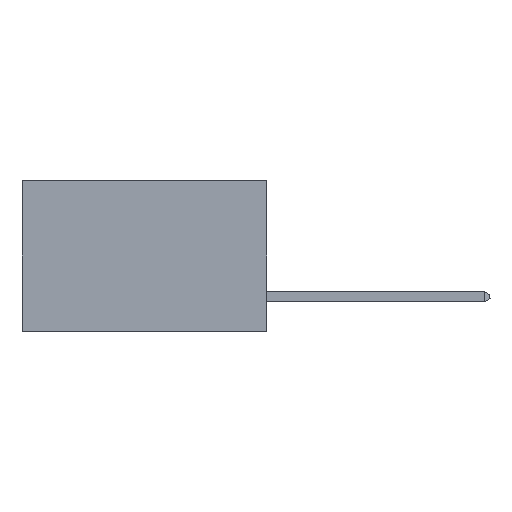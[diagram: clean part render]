
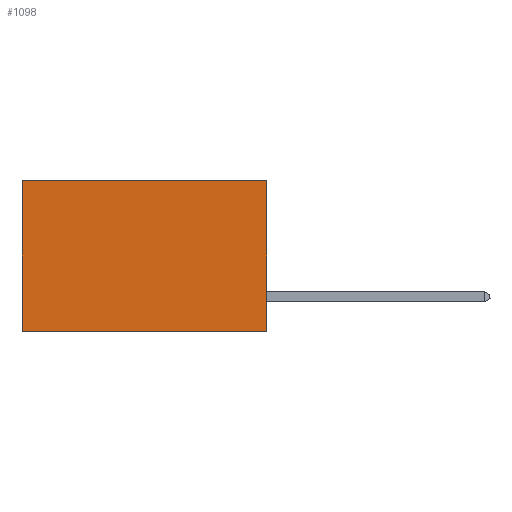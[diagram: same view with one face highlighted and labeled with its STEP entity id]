
A CAD part, left-side view. The second image highlights one B-rep face of the part: STEP entity #1098.
In plain terms, the highlighted planar face has unit normal (-1, 0, 0).
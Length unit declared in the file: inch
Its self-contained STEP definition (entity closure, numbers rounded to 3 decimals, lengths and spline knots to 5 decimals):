
#548 = LINE ( 'NONE', #18708, #14343 ) ;
#1098 = ADVANCED_FACE ( 'NONE', ( #4357 ), #11884, .F. ) ;
#1171 = VERTEX_POINT ( 'NONE', #11953 ) ;
#1679 = EDGE_CURVE ( 'NONE', #11081, #1171, #4578, .T. ) ;
#2158 = CARTESIAN_POINT ( 'NONE',  ( 0.2875, 0., -0.37 ) ) ;
#2663 = VECTOR ( 'NONE', #13475, 39.37008 ) ;
#3350 = VERTEX_POINT ( 'NONE', #3455 ) ;
#3455 = CARTESIAN_POINT ( 'NONE',  ( 0.2875, 0.6, 0. ) ) ;
#3482 = DIRECTION ( 'NONE',  ( 0., 1., 0. ) ) ;
#4357 = FACE_OUTER_BOUND ( 'NONE', #10040, .T. ) ;
#4578 = LINE ( 'NONE', #5097, #11455 ) ;
#5021 = VECTOR ( 'NONE', #8514, 39.37008 ) ;
#5097 = CARTESIAN_POINT ( 'NONE',  ( 0.2875, 0., -0.37 ) ) ;
#6683 = CARTESIAN_POINT ( 'NONE',  ( 0.2875, 0., 0. ) ) ;
#8136 = LINE ( 'NONE', #19115, #5021 ) ;
#8514 = DIRECTION ( 'NONE',  ( 0., 1., 0. ) ) ;
#10040 = EDGE_LOOP ( 'NONE', ( #17172, #18937, #10518, #14161 ) ) ;
#10326 = AXIS2_PLACEMENT_3D ( 'NONE', #10358, #12017, #13566 ) ;
#10358 = CARTESIAN_POINT ( 'NONE',  ( 0.2875, 0., 0. ) ) ;
#10518 = ORIENTED_EDGE ( 'NONE', *, *, #13257, .F. ) ;
#11081 = VERTEX_POINT ( 'NONE', #2158 ) ;
#11455 = VECTOR ( 'NONE', #3482, 39.37008 ) ;
#11884 = PLANE ( 'NONE',  #10326 ) ;
#11953 = CARTESIAN_POINT ( 'NONE',  ( 0.2875, 0.6, -0.37 ) ) ;
#12017 = DIRECTION ( 'NONE',  ( 1., 0., 0. ) ) ;
#12468 = EDGE_CURVE ( 'NONE', #15171, #3350, #8136, .T. ) ;
#13214 = CARTESIAN_POINT ( 'NONE',  ( 0.2875, 0., 0. ) ) ;
#13257 = EDGE_CURVE ( 'NONE', #15171, #11081, #14292, .T. ) ;
#13475 = DIRECTION ( 'NONE',  ( 0., 0., -1. ) ) ;
#13566 = DIRECTION ( 'NONE',  ( 0., 0., -1. ) ) ;
#14161 = ORIENTED_EDGE ( 'NONE', *, *, #12468, .T. ) ;
#14292 = LINE ( 'NONE', #13214, #2663 ) ;
#14343 = VECTOR ( 'NONE', #18891, 39.37008 ) ;
#15171 = VERTEX_POINT ( 'NONE', #6683 ) ;
#17172 = ORIENTED_EDGE ( 'NONE', *, *, #17551, .T. ) ;
#17551 = EDGE_CURVE ( 'NONE', #3350, #1171, #548, .T. ) ;
#18708 = CARTESIAN_POINT ( 'NONE',  ( 0.2875, 0.6, 0. ) ) ;
#18891 = DIRECTION ( 'NONE',  ( 0., 0., -1. ) ) ;
#18937 = ORIENTED_EDGE ( 'NONE', *, *, #1679, .F. ) ;
#19115 = CARTESIAN_POINT ( 'NONE',  ( 0.2875, 0., 0. ) ) ;
